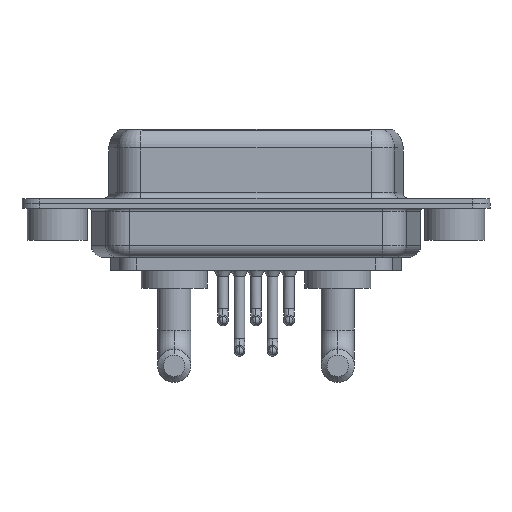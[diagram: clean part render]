
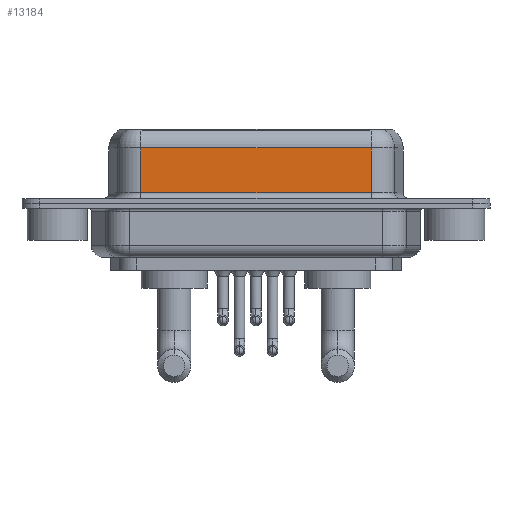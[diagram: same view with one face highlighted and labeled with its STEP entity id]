
A CAD part, front view. The second image highlights one B-rep face of the part: STEP entity #13184.
In plain terms, the highlighted planar face has unit normal (0, -1, 0).
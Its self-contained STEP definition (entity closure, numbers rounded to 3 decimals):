
#20 = CARTESIAN_POINT ( 'NONE',  ( 26.287, -3.95, 6.4 ) ) ;
#345 = PLANE ( 'NONE',  #5824 ) ;
#834 = CARTESIAN_POINT ( 'NONE',  ( 7.013, -3.95, 0.9 ) ) ;
#1162 = CARTESIAN_POINT ( 'NONE',  ( 26.287, -3.95, 6.4 ) ) ;
#1434 = VERTEX_POINT ( 'NONE', #14682 ) ;
#1476 = FACE_OUTER_BOUND ( 'NONE', #14800, .T. ) ;
#1834 = EDGE_CURVE ( 'NONE', #6233, #10488, #4831, .T. ) ;
#1932 = ORIENTED_EDGE ( 'NONE', *, *, #12591, .T. ) ;
#2221 = DIRECTION ( 'NONE',  ( 0., 0., -1. ) ) ;
#3059 = VECTOR ( 'NONE', #3887, 1000. ) ;
#3887 = DIRECTION ( 'NONE',  ( 1., 0., 0. ) ) ;
#4213 = CARTESIAN_POINT ( 'NONE',  ( 26.287, -3.95, 4.65 ) ) ;
#4472 = CARTESIAN_POINT ( 'NONE',  ( 26.287, -3.95, 0.9 ) ) ;
#4774 = CARTESIAN_POINT ( 'NONE',  ( 7.013, -3.95, 6.4 ) ) ;
#4831 = LINE ( 'NONE', #1162, #12344 ) ;
#5824 = AXIS2_PLACEMENT_3D ( 'NONE', #20, #8057, #15625 ) ;
#6233 = VERTEX_POINT ( 'NONE', #4213 ) ;
#6815 = EDGE_CURVE ( 'NONE', #1434, #15234, #8462, .T. ) ;
#8057 = DIRECTION ( 'NONE',  ( 0., 1., 0. ) ) ;
#8366 = ORIENTED_EDGE ( 'NONE', *, *, #1834, .F. ) ;
#8462 = LINE ( 'NONE', #4774, #12199 ) ;
#8680 = ORIENTED_EDGE ( 'NONE', *, *, #14534, .T. ) ;
#9165 = DIRECTION ( 'NONE',  ( -1., 0., 0. ) ) ;
#9338 = VECTOR ( 'NONE', #9165, 1000. ) ;
#10114 = LINE ( 'NONE', #15302, #3059 ) ;
#10488 = VERTEX_POINT ( 'NONE', #4472 ) ;
#10699 = LINE ( 'NONE', #15873, #9338 ) ;
#11326 = DIRECTION ( 'NONE',  ( 0., 0., -1. ) ) ;
#12199 = VECTOR ( 'NONE', #2221, 1000. ) ;
#12331 = ORIENTED_EDGE ( 'NONE', *, *, #6815, .T. ) ;
#12344 = VECTOR ( 'NONE', #11326, 1000. ) ;
#12591 = EDGE_CURVE ( 'NONE', #15234, #10488, #10114, .T. ) ;
#13184 = ADVANCED_FACE ( 'NONE', ( #1476 ), #345, .F. ) ;
#14534 = EDGE_CURVE ( 'NONE', #6233, #1434, #10699, .T. ) ;
#14682 = CARTESIAN_POINT ( 'NONE',  ( 7.013, -3.95, 4.65 ) ) ;
#14800 = EDGE_LOOP ( 'NONE', ( #8366, #8680, #12331, #1932 ) ) ;
#15234 = VERTEX_POINT ( 'NONE', #834 ) ;
#15302 = CARTESIAN_POINT ( 'NONE',  ( 26.287, -3.95, 0.9 ) ) ;
#15625 = DIRECTION ( 'NONE',  ( 0., 0., 1. ) ) ;
#15873 = CARTESIAN_POINT ( 'NONE',  ( 26.287, -3.95, 4.65 ) ) ;
